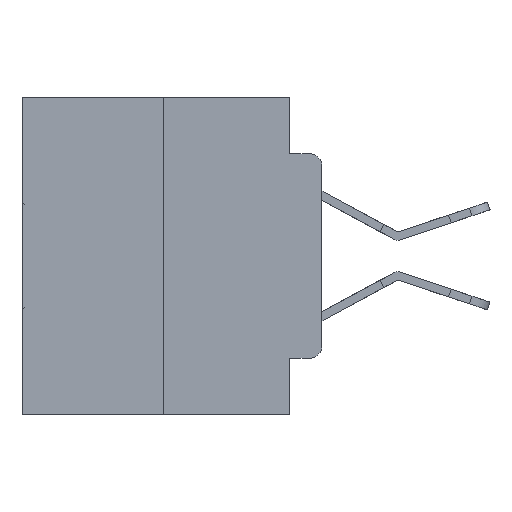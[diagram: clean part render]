
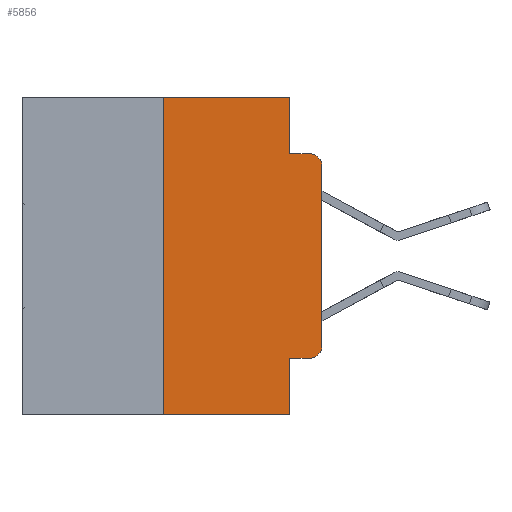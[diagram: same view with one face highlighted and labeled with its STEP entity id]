
A CAD part, left-side view. The second image highlights one B-rep face of the part: STEP entity #5856.
In plain terms, the highlighted planar face has unit normal (-1, 0, 0).
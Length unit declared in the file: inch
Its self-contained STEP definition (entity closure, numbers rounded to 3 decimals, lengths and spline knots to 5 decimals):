
#254 = ORIENTED_EDGE ( 'NONE', *, *, #22773, .F. ) ;
#610 = LINE ( 'NONE', #29552, #6430 ) ;
#813 = ORIENTED_EDGE ( 'NONE', *, *, #18037, .T. ) ;
#973 = ORIENTED_EDGE ( 'NONE', *, *, #12642, .T. ) ;
#1088 = CARTESIAN_POINT ( 'NONE',  ( 0., 0.051, -0.4115 ) ) ;
#1109 = EDGE_LOOP ( 'NONE', ( #813, #2828, #254, #3501, #18792, #14768, #18292, #15959, #13966, #973 ) ) ;
#1517 = AXIS2_PLACEMENT_3D ( 'NONE', #9489, #26017, #11887 ) ;
#2424 = CARTESIAN_POINT ( 'NONE',  ( 0., 0.051, 0. ) ) ;
#2828 = ORIENTED_EDGE ( 'NONE', *, *, #21194, .T. ) ;
#3501 = ORIENTED_EDGE ( 'NONE', *, *, #27486, .F. ) ;
#4215 = DIRECTION ( 'NONE',  ( 0., 0., -1. ) ) ;
#4457 = PLANE ( 'NONE',  #29275 ) ;
#4615 = EDGE_CURVE ( 'NONE', #29319, #13311, #23463, .T. ) ;
#4709 = VECTOR ( 'NONE', #4215, 39.37008 ) ;
#5684 = VECTOR ( 'NONE', #7745, 39.37008 ) ;
#5811 = VERTEX_POINT ( 'NONE', #20957 ) ;
#5856 = ADVANCED_FACE ( 'NONE', ( #15727 ), #4457, .F. ) ;
#6256 = LINE ( 'NONE', #27691, #18178 ) ;
#6398 = VECTOR ( 'NONE', #15586, 39.37008 ) ;
#6407 = CARTESIAN_POINT ( 'NONE',  ( 0., 0.02, -0.0885 ) ) ;
#6430 = VECTOR ( 'NONE', #13006, 39.37008 ) ;
#6917 = DIRECTION ( 'NONE',  ( 0., 0., -1. ) ) ;
#7048 = VERTEX_POINT ( 'NONE', #15931 ) ;
#7233 = CIRCLE ( 'NONE', #1517, 0.02 ) ;
#7745 = DIRECTION ( 'NONE',  ( 0., -1., 0. ) ) ;
#7799 = EDGE_CURVE ( 'NONE', #13311, #17661, #6256, .T. ) ;
#7878 = EDGE_CURVE ( 'NONE', #7048, #28760, #22955, .T. ) ;
#8321 = AXIS2_PLACEMENT_3D ( 'NONE', #25951, #11817, #28355 ) ;
#9275 = CARTESIAN_POINT ( 'NONE',  ( 0., 0.25, -0.5 ) ) ;
#9489 = CARTESIAN_POINT ( 'NONE',  ( 0., 0.02, -0.1085 ) ) ;
#10888 = VECTOR ( 'NONE', #23401, 39.37008 ) ;
#11057 = EDGE_CURVE ( 'NONE', #7048, #5811, #23808, .T. ) ;
#11776 = CARTESIAN_POINT ( 'NONE',  ( 0., 0.25, 0. ) ) ;
#11817 = DIRECTION ( 'NONE',  ( -1., 0., 0. ) ) ;
#11887 = DIRECTION ( 'NONE',  ( 0., 0., -1. ) ) ;
#12642 = EDGE_CURVE ( 'NONE', #5811, #18749, #26616, .T. ) ;
#13006 = DIRECTION ( 'NONE',  ( 0., -1., 0. ) ) ;
#13311 = VERTEX_POINT ( 'NONE', #11776 ) ;
#13966 = ORIENTED_EDGE ( 'NONE', *, *, #11057, .T. ) ;
#14768 = ORIENTED_EDGE ( 'NONE', *, *, #4615, .F. ) ;
#15586 = DIRECTION ( 'NONE',  ( 0., -1., 0. ) ) ;
#15727 = FACE_OUTER_BOUND ( 'NONE', #1109, .T. ) ;
#15931 = CARTESIAN_POINT ( 'NONE',  ( 0., 0.051, -0.4115 ) ) ;
#15959 = ORIENTED_EDGE ( 'NONE', *, *, #7878, .F. ) ;
#16850 = DIRECTION ( 'NONE',  ( 0., 0., -1. ) ) ;
#17650 = CARTESIAN_POINT ( 'NONE',  ( 0., 0., 0. ) ) ;
#17661 = VERTEX_POINT ( 'NONE', #30569 ) ;
#17926 = VECTOR ( 'NONE', #20028, 39.37008 ) ;
#18037 = EDGE_CURVE ( 'NONE', #18749, #28167, #29720, .T. ) ;
#18178 = VECTOR ( 'NONE', #30103, 39.37008 ) ;
#18292 = ORIENTED_EDGE ( 'NONE', *, *, #30865, .T. ) ;
#18749 = VERTEX_POINT ( 'NONE', #27272 ) ;
#18792 = ORIENTED_EDGE ( 'NONE', *, *, #7799, .F. ) ;
#20028 = DIRECTION ( 'NONE',  ( 0., 0., 1. ) ) ;
#20957 = CARTESIAN_POINT ( 'NONE',  ( 0., 0.02, -0.4115 ) ) ;
#21053 = CARTESIAN_POINT ( 'NONE',  ( 0., 0.473, 0. ) ) ;
#21151 = DIRECTION ( 'NONE',  ( 1., 0., 0. ) ) ;
#21194 = EDGE_CURVE ( 'NONE', #28167, #22310, #7233, .T. ) ;
#21956 = CARTESIAN_POINT ( 'NONE',  ( 0., 0.473, -0.5 ) ) ;
#22310 = VERTEX_POINT ( 'NONE', #6407 ) ;
#22773 = EDGE_CURVE ( 'NONE', #23015, #22310, #610, .T. ) ;
#22955 = LINE ( 'NONE', #23258, #4709 ) ;
#23015 = VERTEX_POINT ( 'NONE', #30581 ) ;
#23136 = LINE ( 'NONE', #21956, #5684 ) ;
#23258 = CARTESIAN_POINT ( 'NONE',  ( 0., 0.051, 0. ) ) ;
#23307 = CARTESIAN_POINT ( 'NONE',  ( 0., 0.25, 0. ) ) ;
#23365 = CARTESIAN_POINT ( 'NONE',  ( 0., 0.051, -0.5 ) ) ;
#23401 = DIRECTION ( 'NONE',  ( 0., 0., 1. ) ) ;
#23463 = LINE ( 'NONE', #23307, #10888 ) ;
#23710 = LINE ( 'NONE', #2424, #30014 ) ;
#23808 = LINE ( 'NONE', #1088, #6398 ) ;
#25951 = CARTESIAN_POINT ( 'NONE',  ( 0., 0.02, -0.3915 ) ) ;
#26017 = DIRECTION ( 'NONE',  ( -1., 0., 0. ) ) ;
#26616 = CIRCLE ( 'NONE', #8321, 0.02 ) ;
#27272 = CARTESIAN_POINT ( 'NONE',  ( 0., 0., -0.3915 ) ) ;
#27486 = EDGE_CURVE ( 'NONE', #17661, #23015, #23710, .T. ) ;
#27691 = CARTESIAN_POINT ( 'NONE',  ( 0., 0.473, 0. ) ) ;
#28167 = VERTEX_POINT ( 'NONE', #28549 ) ;
#28355 = DIRECTION ( 'NONE',  ( 0., 0., -1. ) ) ;
#28549 = CARTESIAN_POINT ( 'NONE',  ( 0., 0., -0.1085 ) ) ;
#28760 = VERTEX_POINT ( 'NONE', #23365 ) ;
#29275 = AXIS2_PLACEMENT_3D ( 'NONE', #21053, #21151, #6917 ) ;
#29319 = VERTEX_POINT ( 'NONE', #9275 ) ;
#29552 = CARTESIAN_POINT ( 'NONE',  ( 0., 0.051, -0.0885 ) ) ;
#29720 = LINE ( 'NONE', #17650, #17926 ) ;
#30014 = VECTOR ( 'NONE', #16850, 39.37008 ) ;
#30103 = DIRECTION ( 'NONE',  ( 0., -1., 0. ) ) ;
#30569 = CARTESIAN_POINT ( 'NONE',  ( 0., 0.051, 0. ) ) ;
#30581 = CARTESIAN_POINT ( 'NONE',  ( 0., 0.051, -0.0885 ) ) ;
#30865 = EDGE_CURVE ( 'NONE', #29319, #28760, #23136, .T. ) ;
